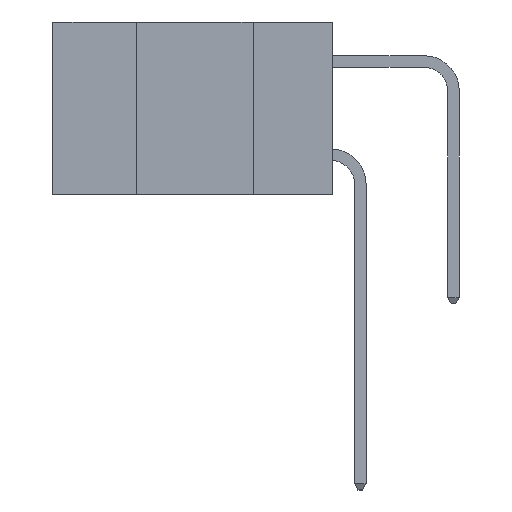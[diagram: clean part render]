
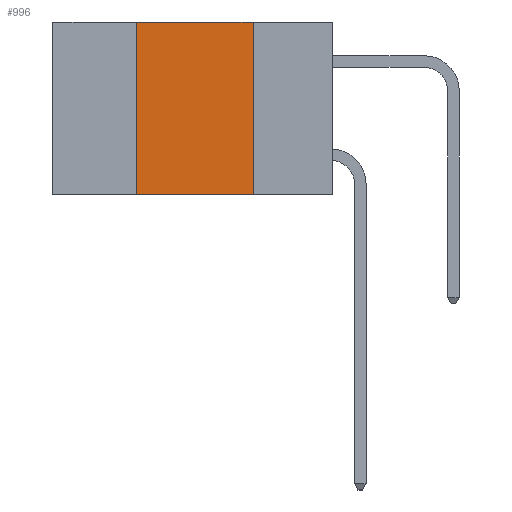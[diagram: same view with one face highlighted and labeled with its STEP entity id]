
A CAD part, left-side view. The second image highlights one B-rep face of the part: STEP entity #996.
In plain terms, the highlighted planar face has unit normal (-1, 0, 0).
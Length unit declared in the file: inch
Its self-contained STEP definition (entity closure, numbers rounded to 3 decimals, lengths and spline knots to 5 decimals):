
#338 = PLANE ( 'NONE',  #13424 ) ;
#480 = CARTESIAN_POINT ( 'NONE',  ( 0., 0.6, 0. ) ) ;
#711 = CARTESIAN_POINT ( 'NONE',  ( 0., 0.42, -0.37 ) ) ;
#996 = ADVANCED_FACE ( 'NONE', ( #11461 ), #338, .F. ) ;
#2078 = VECTOR ( 'NONE', #9286, 39.37008 ) ;
#2498 = LINE ( 'NONE', #10350, #8010 ) ;
#2638 = ORIENTED_EDGE ( 'NONE', *, *, #6610, .T. ) ;
#2970 = VECTOR ( 'NONE', #13358, 39.37008 ) ;
#3201 = VECTOR ( 'NONE', #11666, 39.37008 ) ;
#4354 = ORIENTED_EDGE ( 'NONE', *, *, #13817, .F. ) ;
#4908 = EDGE_LOOP ( 'NONE', ( #4354, #13419, #8692, #2638 ) ) ;
#5014 = LINE ( 'NONE', #9475, #2078 ) ;
#5498 = CARTESIAN_POINT ( 'NONE',  ( 0., 0.42, 0. ) ) ;
#5956 = LINE ( 'NONE', #13468, #2970 ) ;
#6205 = LINE ( 'NONE', #11712, #3201 ) ;
#6610 = EDGE_CURVE ( 'NONE', #11556, #12064, #5956, .T. ) ;
#7829 = CARTESIAN_POINT ( 'NONE',  ( 0., 0.17, 0. ) ) ;
#8010 = VECTOR ( 'NONE', #10335, 39.37008 ) ;
#8389 = VERTEX_POINT ( 'NONE', #5498 ) ;
#8692 = ORIENTED_EDGE ( 'NONE', *, *, #10306, .F. ) ;
#9286 = DIRECTION ( 'NONE',  ( 0., 0., 1. ) ) ;
#9475 = CARTESIAN_POINT ( 'NONE',  ( 0., 0.42, -0.37 ) ) ;
#10306 = EDGE_CURVE ( 'NONE', #11556, #8389, #5014, .T. ) ;
#10335 = DIRECTION ( 'NONE',  ( 0., -1., 0. ) ) ;
#10350 = CARTESIAN_POINT ( 'NONE',  ( 0., 0.6, 0. ) ) ;
#10491 = VERTEX_POINT ( 'NONE', #7829 ) ;
#11461 = FACE_OUTER_BOUND ( 'NONE', #4908, .T. ) ;
#11483 = DIRECTION ( 'NONE',  ( 1., 0., 0. ) ) ;
#11498 = DIRECTION ( 'NONE',  ( 0., 0., -1. ) ) ;
#11556 = VERTEX_POINT ( 'NONE', #711 ) ;
#11666 = DIRECTION ( 'NONE',  ( 0., 0., -1. ) ) ;
#11712 = CARTESIAN_POINT ( 'NONE',  ( 0., 0.17, -0.37 ) ) ;
#12064 = VERTEX_POINT ( 'NONE', #13395 ) ;
#13184 = EDGE_CURVE ( 'NONE', #8389, #10491, #2498, .T. ) ;
#13358 = DIRECTION ( 'NONE',  ( 0., -1., 0. ) ) ;
#13395 = CARTESIAN_POINT ( 'NONE',  ( 0., 0.17, -0.37 ) ) ;
#13419 = ORIENTED_EDGE ( 'NONE', *, *, #13184, .F. ) ;
#13424 = AXIS2_PLACEMENT_3D ( 'NONE', #480, #11483, #11498 ) ;
#13468 = CARTESIAN_POINT ( 'NONE',  ( 0., 0.6, -0.37 ) ) ;
#13817 = EDGE_CURVE ( 'NONE', #10491, #12064, #6205, .T. ) ;
